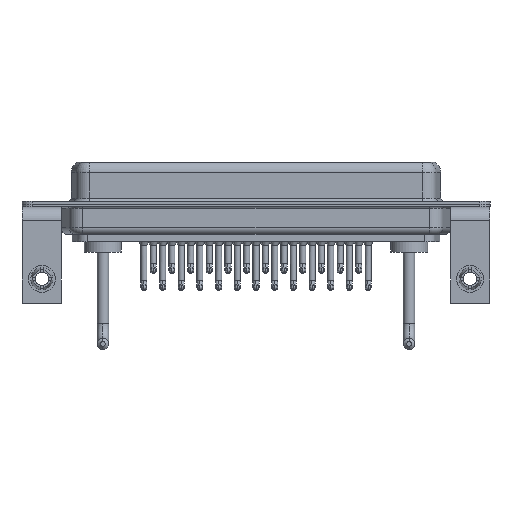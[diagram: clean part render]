
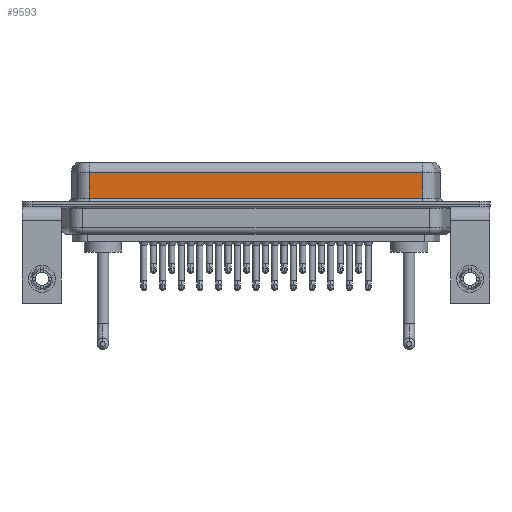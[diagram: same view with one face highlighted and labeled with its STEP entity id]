
A CAD part, front view. The second image highlights one B-rep face of the part: STEP entity #9593.
In plain terms, the highlighted planar face has unit normal (0, -1, 0).
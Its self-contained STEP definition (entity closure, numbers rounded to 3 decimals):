
#137 = EDGE_CURVE ( 'NONE', #1187, #579, #14382, .T. ) ;
#579 = VERTEX_POINT ( 'NONE', #25313 ) ;
#1187 = VERTEX_POINT ( 'NONE', #23652 ) ;
#1845 = CARTESIAN_POINT ( 'NONE',  ( 56.462, -3.95, 4.65 ) ) ;
#2311 = DIRECTION ( 'NONE',  ( 0., 1., 0. ) ) ;
#3039 = VERTEX_POINT ( 'NONE', #1845 ) ;
#4099 = VECTOR ( 'NONE', #8593, 1000. ) ;
#6236 = DIRECTION ( 'NONE',  ( 1., 0., 0. ) ) ;
#6802 = AXIS2_PLACEMENT_3D ( 'NONE', #11019, #2311, #19404 ) ;
#8593 = DIRECTION ( 'NONE',  ( -1., 0., 0. ) ) ;
#8598 = EDGE_CURVE ( 'NONE', #3039, #26690, #14244, .T. ) ;
#9593 = ADVANCED_FACE ( 'NONE', ( #17193 ), #23535, .F. ) ;
#10517 = DIRECTION ( 'NONE',  ( 0., 0., -1. ) ) ;
#11019 = CARTESIAN_POINT ( 'NONE',  ( 56.462, -3.95, 6.4 ) ) ;
#11168 = ORIENTED_EDGE ( 'NONE', *, *, #8598, .T. ) ;
#12448 = CARTESIAN_POINT ( 'NONE',  ( 56.462, -3.95, 4.65 ) ) ;
#13126 = CARTESIAN_POINT ( 'NONE',  ( 7.038, -3.95, 4.65 ) ) ;
#14226 = CARTESIAN_POINT ( 'NONE',  ( 7.038, -3.95, 6.4 ) ) ;
#14244 = LINE ( 'NONE', #12448, #4099 ) ;
#14382 = LINE ( 'NONE', #18659, #21392 ) ;
#14391 = ORIENTED_EDGE ( 'NONE', *, *, #19170, .T. ) ;
#15259 = ORIENTED_EDGE ( 'NONE', *, *, #137, .T. ) ;
#17193 = FACE_OUTER_BOUND ( 'NONE', #17214, .T. ) ;
#17214 = EDGE_LOOP ( 'NONE', ( #26828, #11168, #14391, #15259 ) ) ;
#18659 = CARTESIAN_POINT ( 'NONE',  ( 56.462, -3.95, 0.9 ) ) ;
#19170 = EDGE_CURVE ( 'NONE', #26690, #1187, #21102, .T. ) ;
#19404 = DIRECTION ( 'NONE',  ( 0., 0., 1. ) ) ;
#21102 = LINE ( 'NONE', #14226, #27029 ) ;
#21392 = VECTOR ( 'NONE', #6236, 1000. ) ;
#23535 = PLANE ( 'NONE',  #6802 ) ;
#23652 = CARTESIAN_POINT ( 'NONE',  ( 7.038, -3.95, 0.9 ) ) ;
#24271 = LINE ( 'NONE', #26979, #25029 ) ;
#24762 = EDGE_CURVE ( 'NONE', #3039, #579, #24271, .T. ) ;
#25029 = VECTOR ( 'NONE', #26575, 1000. ) ;
#25313 = CARTESIAN_POINT ( 'NONE',  ( 56.462, -3.95, 0.9 ) ) ;
#26575 = DIRECTION ( 'NONE',  ( 0., 0., -1. ) ) ;
#26690 = VERTEX_POINT ( 'NONE', #13126 ) ;
#26828 = ORIENTED_EDGE ( 'NONE', *, *, #24762, .F. ) ;
#26979 = CARTESIAN_POINT ( 'NONE',  ( 56.462, -3.95, 6.4 ) ) ;
#27029 = VECTOR ( 'NONE', #10517, 1000. ) ;
